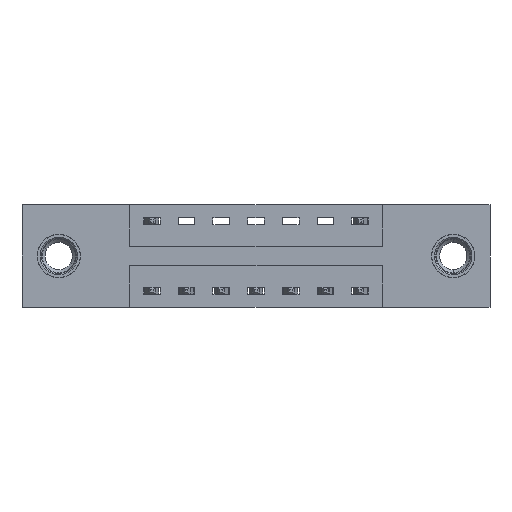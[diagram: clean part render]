
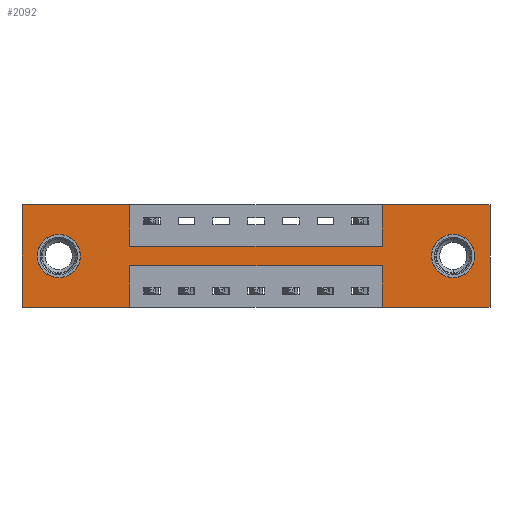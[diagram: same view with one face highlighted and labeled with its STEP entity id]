
A CAD part, front view. The second image highlights one B-rep face of the part: STEP entity #2092.
In plain terms, the highlighted planar face has unit normal (0, -1, 0).
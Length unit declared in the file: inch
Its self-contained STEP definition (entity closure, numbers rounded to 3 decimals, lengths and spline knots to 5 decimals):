
#96 = AXIS2_PLACEMENT_3D ( 'NONE', #4752, #10194, #5566 ) ;
#294 = VECTOR ( 'NONE', #1566, 39.37008 ) ;
#433 = DIRECTION ( 'NONE',  ( -1., 0., 0. ) ) ;
#537 = EDGE_LOOP ( 'NONE', ( #9810, #4555, #1712, #5516, #6016, #2634, #6080, #7883, #2753, #4027, #7491, #9858 ) ) ;
#658 = VECTOR ( 'NONE', #433, 39.37008 ) ;
#680 = EDGE_LOOP ( 'NONE', ( #4536, #6183 ) ) ;
#892 = CARTESIAN_POINT ( 'NONE',  ( 1.685, 0., 0. ) ) ;
#1120 = DIRECTION ( 'NONE',  ( 1., 0., 0. ) ) ;
#1385 = EDGE_CURVE ( 'NONE', #2053, #1440, #10294, .T. ) ;
#1393 = DIRECTION ( 'NONE',  ( 0., 0., 1. ) ) ;
#1407 = DIRECTION ( 'NONE',  ( 0., 1., 0. ) ) ;
#1440 = VERTEX_POINT ( 'NONE', #9941 ) ;
#1447 = VERTEX_POINT ( 'NONE', #6899 ) ;
#1566 = DIRECTION ( 'NONE',  ( -1., 0., 0. ) ) ;
#1627 = EDGE_CURVE ( 'NONE', #6315, #10108, #1779, .T. ) ;
#1664 = CARTESIAN_POINT ( 'NONE',  ( 0.3875, 0., 0. ) ) ;
#1712 = ORIENTED_EDGE ( 'NONE', *, *, #8888, .F. ) ;
#1779 = CIRCLE ( 'NONE', #96, 0.078 ) ;
#1781 = EDGE_CURVE ( 'NONE', #2064, #6110, #6964, .T. ) ;
#1886 = VERTEX_POINT ( 'NONE', #3459 ) ;
#1915 = VECTOR ( 'NONE', #1120, 39.37008 ) ;
#1962 = VECTOR ( 'NONE', #2282, 39.37008 ) ;
#2053 = VERTEX_POINT ( 'NONE', #9970 ) ;
#2064 = VERTEX_POINT ( 'NONE', #4491 ) ;
#2092 = ADVANCED_FACE ( 'NONE', ( #3767, #8020, #8238 ), #7786, .T. ) ;
#2093 = VECTOR ( 'NONE', #2466, 39.37008 ) ;
#2228 = CARTESIAN_POINT ( 'NONE',  ( 0., 0., 0. ) ) ;
#2274 = EDGE_CURVE ( 'NONE', #10108, #6315, #3624, .T. ) ;
#2282 = DIRECTION ( 'NONE',  ( -1., 0., 0. ) ) ;
#2352 = VECTOR ( 'NONE', #6501, 39.37008 ) ;
#2401 = VERTEX_POINT ( 'NONE', #7710 ) ;
#2466 = DIRECTION ( 'NONE',  ( 0., 0., -1. ) ) ;
#2488 = LINE ( 'NONE', #3984, #294 ) ;
#2496 = VECTOR ( 'NONE', #4194, 39.37008 ) ;
#2595 = CARTESIAN_POINT ( 'NONE',  ( 0.3875, 0., -0.22 ) ) ;
#2634 = ORIENTED_EDGE ( 'NONE', *, *, #1385, .F. ) ;
#2753 = ORIENTED_EDGE ( 'NONE', *, *, #8971, .F. ) ;
#2946 = CARTESIAN_POINT ( 'NONE',  ( 1.685, 0., -0.37 ) ) ;
#2959 = DIRECTION ( 'NONE',  ( 0., -1., 0. ) ) ;
#3252 = CARTESIAN_POINT ( 'NONE',  ( 1.2975, 0., 0. ) ) ;
#3262 = ORIENTED_EDGE ( 'NONE', *, *, #8420, .T. ) ;
#3361 = VERTEX_POINT ( 'NONE', #2946 ) ;
#3384 = ORIENTED_EDGE ( 'NONE', *, *, #3561, .T. ) ;
#3459 = CARTESIAN_POINT ( 'NONE',  ( 0.3875, 0., -0.37 ) ) ;
#3561 = EDGE_CURVE ( 'NONE', #9801, #3874, #3593, .T. ) ;
#3593 = CIRCLE ( 'NONE', #4935, 0.078 ) ;
#3624 = CIRCLE ( 'NONE', #4134, 0.078 ) ;
#3767 = FACE_BOUND ( 'NONE', #4544, .T. ) ;
#3874 = VERTEX_POINT ( 'NONE', #5308 ) ;
#3984 = CARTESIAN_POINT ( 'NONE',  ( 0., 0., -0.37 ) ) ;
#4027 = ORIENTED_EDGE ( 'NONE', *, *, #1781, .F. ) ;
#4051 = DIRECTION ( 'NONE',  ( 0., 1., 0. ) ) ;
#4134 = AXIS2_PLACEMENT_3D ( 'NONE', #8996, #4275, #9762 ) ;
#4194 = DIRECTION ( 'NONE',  ( 0., 0., -1. ) ) ;
#4275 = DIRECTION ( 'NONE',  ( 0., 1., 0. ) ) ;
#4334 = CARTESIAN_POINT ( 'NONE',  ( 1.5525, 0., -0.263 ) ) ;
#4489 = LINE ( 'NONE', #9572, #8453 ) ;
#4491 = CARTESIAN_POINT ( 'NONE',  ( 0., 0., 0. ) ) ;
#4536 = ORIENTED_EDGE ( 'NONE', *, *, #1627, .T. ) ;
#4544 = EDGE_LOOP ( 'NONE', ( #3262, #3384 ) ) ;
#4555 = ORIENTED_EDGE ( 'NONE', *, *, #8723, .F. ) ;
#4670 = DIRECTION ( 'NONE',  ( 0., 0., -1. ) ) ;
#4747 = LINE ( 'NONE', #3252, #2352 ) ;
#4752 = CARTESIAN_POINT ( 'NONE',  ( 0.1325, 0., -0.185 ) ) ;
#4881 = CARTESIAN_POINT ( 'NONE',  ( 1.2975, 0., -0.37 ) ) ;
#4935 = AXIS2_PLACEMENT_3D ( 'NONE', #8798, #4051, #9560 ) ;
#5170 = LINE ( 'NONE', #892, #2496 ) ;
#5308 = CARTESIAN_POINT ( 'NONE',  ( 1.5525, 0., -0.107 ) ) ;
#5373 = CARTESIAN_POINT ( 'NONE',  ( 0., 0., -0.37 ) ) ;
#5431 = CARTESIAN_POINT ( 'NONE',  ( 0.1325, 0., -0.263 ) ) ;
#5491 = CARTESIAN_POINT ( 'NONE',  ( 0.3875, 0., -0.37 ) ) ;
#5516 = ORIENTED_EDGE ( 'NONE', *, *, #7955, .F. ) ;
#5566 = DIRECTION ( 'NONE',  ( 0., 0., 1. ) ) ;
#6016 = ORIENTED_EDGE ( 'NONE', *, *, #7482, .F. ) ;
#6049 = AXIS2_PLACEMENT_3D ( 'NONE', #6259, #1407, #7052 ) ;
#6068 = VERTEX_POINT ( 'NONE', #2595 ) ;
#6080 = ORIENTED_EDGE ( 'NONE', *, *, #8905, .F. ) ;
#6110 = VERTEX_POINT ( 'NONE', #8234 ) ;
#6153 = CARTESIAN_POINT ( 'NONE',  ( 0., 0., -0.37 ) ) ;
#6183 = ORIENTED_EDGE ( 'NONE', *, *, #2274, .T. ) ;
#6259 = CARTESIAN_POINT ( 'NONE',  ( 1.5525, 0., -0.185 ) ) ;
#6315 = VERTEX_POINT ( 'NONE', #6992 ) ;
#6389 = LINE ( 'NONE', #1664, #2093 ) ;
#6482 = AXIS2_PLACEMENT_3D ( 'NONE', #5373, #2959, #8548 ) ;
#6501 = DIRECTION ( 'NONE',  ( 0., 0., 1. ) ) ;
#6507 = LINE ( 'NONE', #5491, #8329 ) ;
#6899 = CARTESIAN_POINT ( 'NONE',  ( 1.2975, 0., -0.22 ) ) ;
#6964 = LINE ( 'NONE', #9613, #8677 ) ;
#6992 = CARTESIAN_POINT ( 'NONE',  ( 0.1325, 0., -0.107 ) ) ;
#7052 = DIRECTION ( 'NONE',  ( 0., 0., -1. ) ) ;
#7093 = CARTESIAN_POINT ( 'NONE',  ( 0.3875, 0., -0.22 ) ) ;
#7161 = EDGE_CURVE ( 'NONE', #10328, #2064, #7425, .T. ) ;
#7425 = LINE ( 'NONE', #2228, #9476 ) ;
#7482 = EDGE_CURVE ( 'NONE', #1440, #3361, #5170, .T. ) ;
#7491 = ORIENTED_EDGE ( 'NONE', *, *, #7161, .F. ) ;
#7593 = CARTESIAN_POINT ( 'NONE',  ( 0., 0., 0. ) ) ;
#7710 = CARTESIAN_POINT ( 'NONE',  ( 1.2975, 0., -0.37 ) ) ;
#7786 = PLANE ( 'NONE',  #6482 ) ;
#7883 = ORIENTED_EDGE ( 'NONE', *, *, #8931, .F. ) ;
#7955 = EDGE_CURVE ( 'NONE', #3361, #2401, #2488, .T. ) ;
#8020 = FACE_BOUND ( 'NONE', #680, .T. ) ;
#8078 = DIRECTION ( 'NONE',  ( 1., 0., 0. ) ) ;
#8213 = CIRCLE ( 'NONE', #6049, 0.078 ) ;
#8234 = CARTESIAN_POINT ( 'NONE',  ( 0.3875, 0., 0. ) ) ;
#8238 = FACE_OUTER_BOUND ( 'NONE', #537, .T. ) ;
#8329 = VECTOR ( 'NONE', #4670, 39.37008 ) ;
#8370 = EDGE_CURVE ( 'NONE', #1886, #10328, #8941, .T. ) ;
#8420 = EDGE_CURVE ( 'NONE', #3874, #9801, #8213, .T. ) ;
#8453 = VECTOR ( 'NONE', #8078, 39.37008 ) ;
#8548 = DIRECTION ( 'NONE',  ( 0., 0., -1. ) ) ;
#8677 = VECTOR ( 'NONE', #10316, 39.37008 ) ;
#8703 = LINE ( 'NONE', #4881, #8928 ) ;
#8708 = EDGE_CURVE ( 'NONE', #6068, #1886, #6507, .T. ) ;
#8723 = EDGE_CURVE ( 'NONE', #1447, #6068, #10336, .T. ) ;
#8742 = VERTEX_POINT ( 'NONE', #10154 ) ;
#8760 = CARTESIAN_POINT ( 'NONE',  ( 0., 0., -0.37 ) ) ;
#8798 = CARTESIAN_POINT ( 'NONE',  ( 1.5525, 0., -0.185 ) ) ;
#8888 = EDGE_CURVE ( 'NONE', #2401, #1447, #8703, .T. ) ;
#8905 = EDGE_CURVE ( 'NONE', #8742, #2053, #4747, .T. ) ;
#8928 = VECTOR ( 'NONE', #10308, 39.37008 ) ;
#8931 = EDGE_CURVE ( 'NONE', #9220, #8742, #4489, .T. ) ;
#8941 = LINE ( 'NONE', #6153, #658 ) ;
#8971 = EDGE_CURVE ( 'NONE', #6110, #9220, #6389, .T. ) ;
#8996 = CARTESIAN_POINT ( 'NONE',  ( 0.1325, 0., -0.185 ) ) ;
#9134 = CARTESIAN_POINT ( 'NONE',  ( 0.3875, 0., -0.15 ) ) ;
#9220 = VERTEX_POINT ( 'NONE', #9134 ) ;
#9476 = VECTOR ( 'NONE', #1393, 39.37008 ) ;
#9560 = DIRECTION ( 'NONE',  ( 0., 0., -1. ) ) ;
#9572 = CARTESIAN_POINT ( 'NONE',  ( 0.3875, 0., -0.15 ) ) ;
#9613 = CARTESIAN_POINT ( 'NONE',  ( 0., 0., 0. ) ) ;
#9762 = DIRECTION ( 'NONE',  ( 0., 0., 1. ) ) ;
#9801 = VERTEX_POINT ( 'NONE', #4334 ) ;
#9810 = ORIENTED_EDGE ( 'NONE', *, *, #8708, .F. ) ;
#9858 = ORIENTED_EDGE ( 'NONE', *, *, #8370, .F. ) ;
#9941 = CARTESIAN_POINT ( 'NONE',  ( 1.685, 0., 0. ) ) ;
#9970 = CARTESIAN_POINT ( 'NONE',  ( 1.2975, 0., 0. ) ) ;
#10108 = VERTEX_POINT ( 'NONE', #5431 ) ;
#10154 = CARTESIAN_POINT ( 'NONE',  ( 1.2975, 0., -0.15 ) ) ;
#10194 = DIRECTION ( 'NONE',  ( 0., 1., 0. ) ) ;
#10294 = LINE ( 'NONE', #7593, #1915 ) ;
#10308 = DIRECTION ( 'NONE',  ( 0., 0., 1. ) ) ;
#10316 = DIRECTION ( 'NONE',  ( 1., 0., 0. ) ) ;
#10328 = VERTEX_POINT ( 'NONE', #8760 ) ;
#10336 = LINE ( 'NONE', #7093, #1962 ) ;
